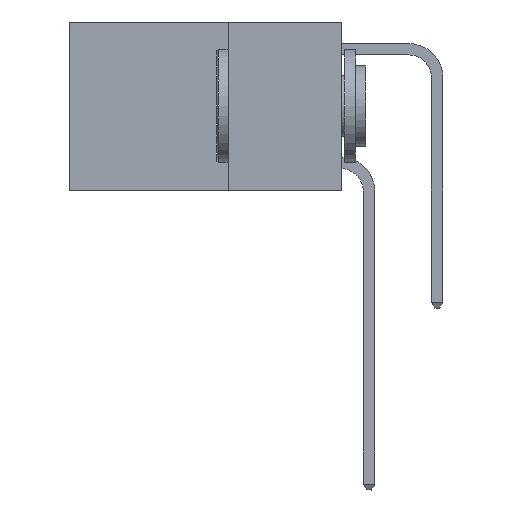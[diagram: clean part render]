
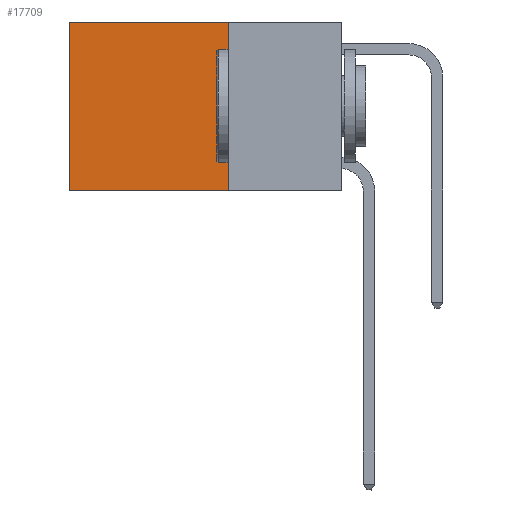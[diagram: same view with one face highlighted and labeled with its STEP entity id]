
A CAD part, left-side view. The second image highlights one B-rep face of the part: STEP entity #17709.
In plain terms, the highlighted planar face has unit normal (-1, 0, 0).
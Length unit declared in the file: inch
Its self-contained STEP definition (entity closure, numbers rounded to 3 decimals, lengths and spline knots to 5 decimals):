
#38 = PLANE ( 'NONE',  #13264 ) ;
#392 = CARTESIAN_POINT ( 'NONE',  ( 0.2625, 0.25, -0.37 ) ) ;
#593 = LINE ( 'NONE', #3020, #12477 ) ;
#857 = VECTOR ( 'NONE', #10128, 39.37008 ) ;
#962 = ORIENTED_EDGE ( 'NONE', *, *, #2894, .F. ) ;
#1872 = EDGE_LOOP ( 'NONE', ( #5302, #7493, #962, #17297 ) ) ;
#2468 = VERTEX_POINT ( 'NONE', #5221 ) ;
#2604 = EDGE_CURVE ( 'NONE', #6089, #17666, #7426, .T. ) ;
#2819 = LINE ( 'NONE', #19516, #13689 ) ;
#2894 = EDGE_CURVE ( 'NONE', #2468, #6089, #2819, .T. ) ;
#3020 = CARTESIAN_POINT ( 'NONE',  ( 0.2625, 0.25, 0. ) ) ;
#5221 = CARTESIAN_POINT ( 'NONE',  ( 0.2625, 0.25, 0. ) ) ;
#5302 = ORIENTED_EDGE ( 'NONE', *, *, #11185, .T. ) ;
#6089 = VERTEX_POINT ( 'NONE', #392 ) ;
#6661 = DIRECTION ( 'NONE',  ( 0., 0., -1. ) ) ;
#7422 = FACE_OUTER_BOUND ( 'NONE', #1872, .T. ) ;
#7426 = LINE ( 'NONE', #15731, #857 ) ;
#7493 = ORIENTED_EDGE ( 'NONE', *, *, #2604, .F. ) ;
#7550 = CARTESIAN_POINT ( 'NONE',  ( 0.2625, 0.6, 0. ) ) ;
#7687 = VERTEX_POINT ( 'NONE', #19771 ) ;
#9220 = DIRECTION ( 'NONE',  ( 0., 1., 0. ) ) ;
#9518 = DIRECTION ( 'NONE',  ( 0., 0., -1. ) ) ;
#9838 = LINE ( 'NONE', #7550, #18712 ) ;
#10128 = DIRECTION ( 'NONE',  ( 0., 1., 0. ) ) ;
#10536 = EDGE_CURVE ( 'NONE', #2468, #7687, #593, .T. ) ;
#11185 = EDGE_CURVE ( 'NONE', #7687, #17666, #9838, .T. ) ;
#12254 = CARTESIAN_POINT ( 'NONE',  ( 0.2625, 0.6, -0.37 ) ) ;
#12477 = VECTOR ( 'NONE', #9220, 39.37008 ) ;
#13264 = AXIS2_PLACEMENT_3D ( 'NONE', #14080, #15453, #9518 ) ;
#13689 = VECTOR ( 'NONE', #15317, 39.37008 ) ;
#14080 = CARTESIAN_POINT ( 'NONE',  ( 0.2625, 0.25, 0. ) ) ;
#15317 = DIRECTION ( 'NONE',  ( 0., 0., -1. ) ) ;
#15453 = DIRECTION ( 'NONE',  ( 1., 0., 0. ) ) ;
#15731 = CARTESIAN_POINT ( 'NONE',  ( 0.2625, 0.25, -0.37 ) ) ;
#17297 = ORIENTED_EDGE ( 'NONE', *, *, #10536, .T. ) ;
#17666 = VERTEX_POINT ( 'NONE', #12254 ) ;
#17709 = ADVANCED_FACE ( 'NONE', ( #7422 ), #38, .F. ) ;
#18712 = VECTOR ( 'NONE', #6661, 39.37008 ) ;
#19516 = CARTESIAN_POINT ( 'NONE',  ( 0.2625, 0.25, 0. ) ) ;
#19771 = CARTESIAN_POINT ( 'NONE',  ( 0.2625, 0.6, 0. ) ) ;
